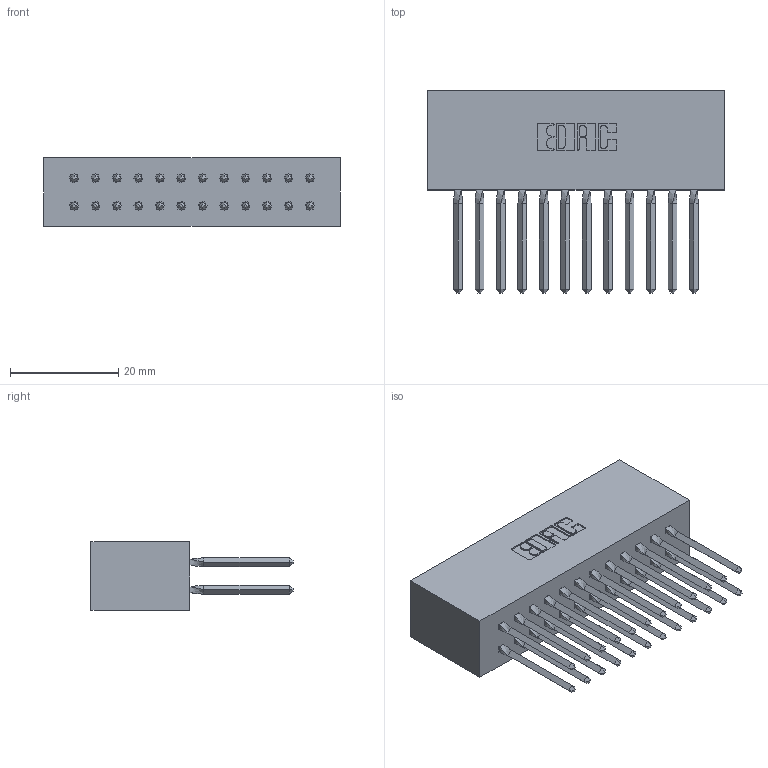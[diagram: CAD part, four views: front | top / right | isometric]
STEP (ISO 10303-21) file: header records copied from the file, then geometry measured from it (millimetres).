
FILE_DESCRIPTION (( 'STEP AP203' ), '1' );
FILE_NAME ('317-024-540-801.STEP', '2020-02-27T18:03:20', ( '' ), ( '' ), 'SwSTEP 2.0', 'SolidWorks 2016', '' );
FILE_SCHEMA (( 'CONFIG_CONTROL_DESIGN' ));
Length unit declared in the file: inch
Products named in the file (3): 317 Part_Lugless; 317-024-540-801; 317-290-001_540
Assembly tree (25 placements, depth 2):
  317-024-540-801
    317 Part_Lugless
    317-290-001_540  x24
Bounding box: 54.76 x 37.34 x 12.7 mm (x, y, z)
Volume: 9970.1 mm3; surface area: 13988 mm2
Topology: 25 solids, 25 shells, 2226 faces, 6167 edges, 3974 vertices
Faces by surface type: plane 1802, cylinder 328, bspline 96
Entity records: 21122 total; most frequent: CARTESIAN_POINT 4095, ORIENTED_EDGE 3594, DIRECTION 2995, EDGE_CURVE 1797, LINE 1549, VECTOR 1549, VERTEX_POINT 1191, AXIS2_PLACEMENT_3D 723
